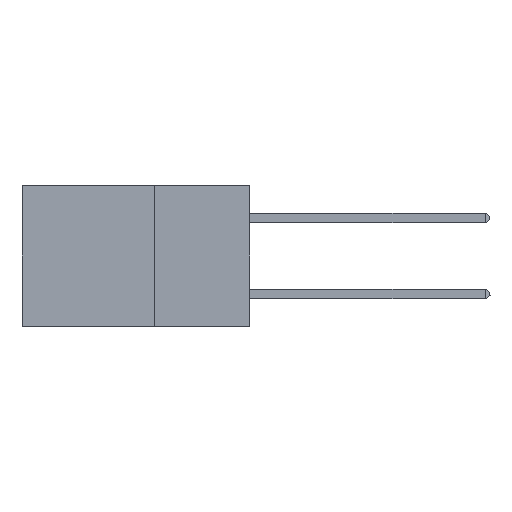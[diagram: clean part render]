
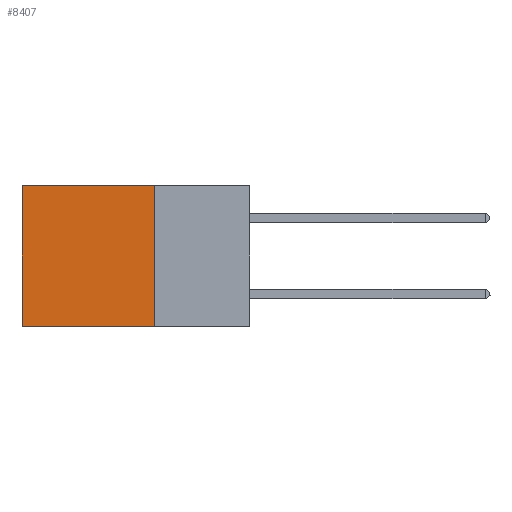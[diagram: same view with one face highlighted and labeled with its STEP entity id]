
A CAD part, left-side view. The second image highlights one B-rep face of the part: STEP entity #8407.
In plain terms, the highlighted planar face has unit normal (-1, 0, 0).
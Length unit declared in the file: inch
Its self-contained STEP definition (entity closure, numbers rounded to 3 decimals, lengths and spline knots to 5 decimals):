
#444 = VERTEX_POINT ( 'NONE', #5024 ) ;
#886 = CARTESIAN_POINT ( 'NONE',  ( 0.2875, 0.25, -0.37 ) ) ;
#1051 = LINE ( 'NONE', #2335, #6975 ) ;
#1861 = CARTESIAN_POINT ( 'NONE',  ( 0.2875, 0.6, -0.37 ) ) ;
#2273 = CARTESIAN_POINT ( 'NONE',  ( 0.2875, 0.6, 0. ) ) ;
#2335 = CARTESIAN_POINT ( 'NONE',  ( 0.2875, 0.25, 0. ) ) ;
#2759 = VECTOR ( 'NONE', #9598, 39.37008 ) ;
#3088 = DIRECTION ( 'NONE',  ( 0., 1., 0. ) ) ;
#3190 = EDGE_CURVE ( 'NONE', #444, #5660, #15236, .T. ) ;
#3517 = VECTOR ( 'NONE', #3088, 39.37008 ) ;
#3612 = CARTESIAN_POINT ( 'NONE',  ( 0.2875, 0.6, 0. ) ) ;
#3674 = FACE_OUTER_BOUND ( 'NONE', #15001, .T. ) ;
#4191 = CARTESIAN_POINT ( 'NONE',  ( 0.2875, 0.25, 0. ) ) ;
#4510 = DIRECTION ( 'NONE',  ( 0., 1., 0. ) ) ;
#5024 = CARTESIAN_POINT ( 'NONE',  ( 0.2875, 0.25, 0. ) ) ;
#5360 = DIRECTION ( 'NONE',  ( 1., 0., 0. ) ) ;
#5660 = VERTEX_POINT ( 'NONE', #3612 ) ;
#6026 = CARTESIAN_POINT ( 'NONE',  ( 0.2875, 0.25, 0. ) ) ;
#6975 = VECTOR ( 'NONE', #7085, 39.37008 ) ;
#6988 = LINE ( 'NONE', #2273, #2759 ) ;
#7085 = DIRECTION ( 'NONE',  ( 0., 0., -1. ) ) ;
#8135 = AXIS2_PLACEMENT_3D ( 'NONE', #4191, #5360, #13727 ) ;
#8407 = ADVANCED_FACE ( 'NONE', ( #3674 ), #10271, .F. ) ;
#8811 = ORIENTED_EDGE ( 'NONE', *, *, #3190, .T. ) ;
#9464 = VECTOR ( 'NONE', #4510, 39.37008 ) ;
#9598 = DIRECTION ( 'NONE',  ( 0., 0., -1. ) ) ;
#9693 = VERTEX_POINT ( 'NONE', #886 ) ;
#9879 = ORIENTED_EDGE ( 'NONE', *, *, #11868, .T. ) ;
#10271 = PLANE ( 'NONE',  #8135 ) ;
#10474 = CARTESIAN_POINT ( 'NONE',  ( 0.2875, 0.25, -0.37 ) ) ;
#10700 = ORIENTED_EDGE ( 'NONE', *, *, #12274, .F. ) ;
#10980 = EDGE_CURVE ( 'NONE', #9693, #15413, #13216, .T. ) ;
#11868 = EDGE_CURVE ( 'NONE', #5660, #15413, #6988, .T. ) ;
#12274 = EDGE_CURVE ( 'NONE', #444, #9693, #1051, .T. ) ;
#13216 = LINE ( 'NONE', #10474, #9464 ) ;
#13727 = DIRECTION ( 'NONE',  ( 0., 0., -1. ) ) ;
#14506 = ORIENTED_EDGE ( 'NONE', *, *, #10980, .F. ) ;
#15001 = EDGE_LOOP ( 'NONE', ( #9879, #14506, #10700, #8811 ) ) ;
#15236 = LINE ( 'NONE', #6026, #3517 ) ;
#15413 = VERTEX_POINT ( 'NONE', #1861 ) ;
